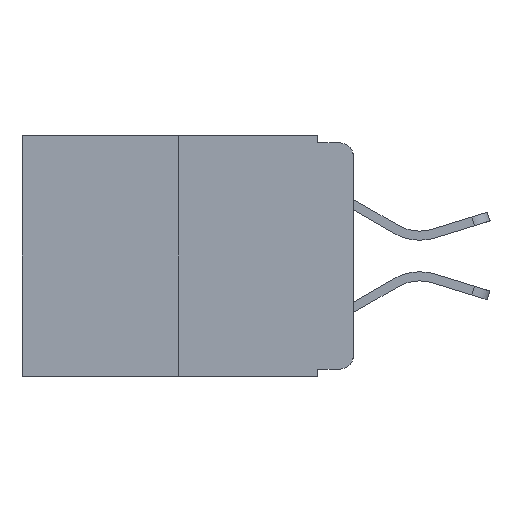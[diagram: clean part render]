
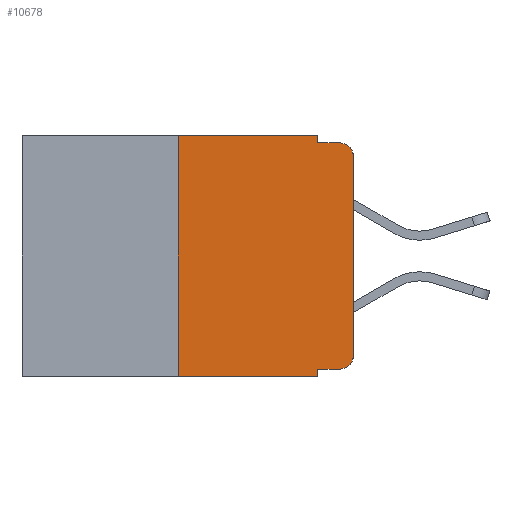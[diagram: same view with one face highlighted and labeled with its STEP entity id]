
A CAD part, left-side view. The second image highlights one B-rep face of the part: STEP entity #10678.
In plain terms, the highlighted planar face has unit normal (-1, 0, 0).
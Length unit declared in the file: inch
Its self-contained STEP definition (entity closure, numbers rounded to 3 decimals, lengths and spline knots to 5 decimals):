
#51 = ORIENTED_EDGE ( 'NONE', *, *, #3855, .T. ) ;
#233 = CARTESIAN_POINT ( 'NONE',  ( 0., 0.25, 0. ) ) ;
#453 = DIRECTION ( 'NONE',  ( -1., 0., 0. ) ) ;
#461 = VECTOR ( 'NONE', #6910, 39.37008 ) ;
#1703 = VECTOR ( 'NONE', #13378, 39.37008 ) ;
#1910 = CARTESIAN_POINT ( 'NONE',  ( 0., 0.051, 0. ) ) ;
#2035 = CARTESIAN_POINT ( 'NONE',  ( 0., 0.051, -0.333 ) ) ;
#2310 = VERTEX_POINT ( 'NONE', #12257 ) ;
#2331 = ORIENTED_EDGE ( 'NONE', *, *, #18353, .F. ) ;
#2452 = VERTEX_POINT ( 'NONE', #16747 ) ;
#2544 = ORIENTED_EDGE ( 'NONE', *, *, #15218, .F. ) ;
#2685 = EDGE_CURVE ( 'NONE', #2310, #16039, #17620, .T. ) ;
#2820 = CARTESIAN_POINT ( 'NONE',  ( 0., 0.25, -0.343 ) ) ;
#2927 = CARTESIAN_POINT ( 'NONE',  ( 0., 0.051, 0. ) ) ;
#3038 = DIRECTION ( 'NONE',  ( 0., 0., -1. ) ) ;
#3256 = ORIENTED_EDGE ( 'NONE', *, *, #7961, .T. ) ;
#3326 = AXIS2_PLACEMENT_3D ( 'NONE', #13756, #5247, #15170 ) ;
#3532 = LINE ( 'NONE', #233, #14521 ) ;
#3755 = ORIENTED_EDGE ( 'NONE', *, *, #10167, .T. ) ;
#3855 = EDGE_CURVE ( 'NONE', #5037, #9958, #14087, .T. ) ;
#3957 = ORIENTED_EDGE ( 'NONE', *, *, #10446, .F. ) ;
#4077 = EDGE_CURVE ( 'NONE', #9958, #2452, #10511, .T. ) ;
#4297 = FACE_OUTER_BOUND ( 'NONE', #16642, .T. ) ;
#4367 = CARTESIAN_POINT ( 'NONE',  ( 0., 0., -0.313 ) ) ;
#4392 = CARTESIAN_POINT ( 'NONE',  ( 0., 0.051, -0.333 ) ) ;
#4405 = ORIENTED_EDGE ( 'NONE', *, *, #6664, .F. ) ;
#4444 = DIRECTION ( 'NONE',  ( 0., 0., -1. ) ) ;
#4838 = CARTESIAN_POINT ( 'NONE',  ( 0., 0.473, -0.343 ) ) ;
#5037 = VERTEX_POINT ( 'NONE', #15895 ) ;
#5043 = LINE ( 'NONE', #18194, #461 ) ;
#5051 = LINE ( 'NONE', #14589, #12199 ) ;
#5247 = DIRECTION ( 'NONE',  ( -1., 0., 0. ) ) ;
#5394 = VERTEX_POINT ( 'NONE', #8325 ) ;
#5466 = CARTESIAN_POINT ( 'NONE',  ( 0., 0., 0. ) ) ;
#6664 = EDGE_CURVE ( 'NONE', #16112, #14730, #3532, .T. ) ;
#6910 = DIRECTION ( 'NONE',  ( 0., -1., 0. ) ) ;
#7139 = VERTEX_POINT ( 'NONE', #4392 ) ;
#7174 = AXIS2_PLACEMENT_3D ( 'NONE', #18675, #11700, #3038 ) ;
#7441 = AXIS2_PLACEMENT_3D ( 'NONE', #9296, #453, #10756 ) ;
#7761 = DIRECTION ( 'NONE',  ( 0., 0., 1. ) ) ;
#7961 = EDGE_CURVE ( 'NONE', #2452, #5394, #12495, .T. ) ;
#8060 = VERTEX_POINT ( 'NONE', #16728 ) ;
#8305 = DIRECTION ( 'NONE',  ( 0., 0., 1. ) ) ;
#8325 = CARTESIAN_POINT ( 'NONE',  ( 0., 0.02, -0.01 ) ) ;
#9296 = CARTESIAN_POINT ( 'NONE',  ( 0., 0.02, -0.313 ) ) ;
#9376 = ORIENTED_EDGE ( 'NONE', *, *, #2685, .F. ) ;
#9576 = VECTOR ( 'NONE', #12102, 39.37008 ) ;
#9850 = ORIENTED_EDGE ( 'NONE', *, *, #4077, .T. ) ;
#9958 = VERTEX_POINT ( 'NONE', #4367 ) ;
#10167 = EDGE_CURVE ( 'NONE', #16112, #8060, #13284, .T. ) ;
#10241 = PLANE ( 'NONE',  #7174 ) ;
#10446 = EDGE_CURVE ( 'NONE', #14730, #2310, #5043, .T. ) ;
#10511 = LINE ( 'NONE', #5466, #17567 ) ;
#10568 = VECTOR ( 'NONE', #4444, 39.37008 ) ;
#10678 = ADVANCED_FACE ( 'NONE', ( #4297 ), #10241, .F. ) ;
#10756 = DIRECTION ( 'NONE',  ( 0., 0., -1. ) ) ;
#11700 = DIRECTION ( 'NONE',  ( 1., 0., 0. ) ) ;
#11753 = DIRECTION ( 'NONE',  ( 0., -1., 0. ) ) ;
#12102 = DIRECTION ( 'NONE',  ( 0., 0., -1. ) ) ;
#12199 = VECTOR ( 'NONE', #11753, 39.37008 ) ;
#12223 = DIRECTION ( 'NONE',  ( 0., -1., 0. ) ) ;
#12257 = CARTESIAN_POINT ( 'NONE',  ( 0., 0.051, 0. ) ) ;
#12495 = CIRCLE ( 'NONE', #3326, 0.02 ) ;
#12933 = LINE ( 'NONE', #1910, #9576 ) ;
#13077 = VECTOR ( 'NONE', #12223, 39.37008 ) ;
#13284 = LINE ( 'NONE', #4838, #1703 ) ;
#13378 = DIRECTION ( 'NONE',  ( 0., -1., 0. ) ) ;
#13756 = CARTESIAN_POINT ( 'NONE',  ( 0., 0.02, -0.03 ) ) ;
#13778 = CARTESIAN_POINT ( 'NONE',  ( 0., 0.25, 0. ) ) ;
#13858 = ORIENTED_EDGE ( 'NONE', *, *, #17907, .T. ) ;
#14087 = CIRCLE ( 'NONE', #7441, 0.02 ) ;
#14159 = CARTESIAN_POINT ( 'NONE',  ( 0., 0.051, -0.01 ) ) ;
#14521 = VECTOR ( 'NONE', #7761, 39.37008 ) ;
#14589 = CARTESIAN_POINT ( 'NONE',  ( 0., 0.051, -0.01 ) ) ;
#14730 = VERTEX_POINT ( 'NONE', #13778 ) ;
#15170 = DIRECTION ( 'NONE',  ( 0., 0., -1. ) ) ;
#15218 = EDGE_CURVE ( 'NONE', #7139, #8060, #12933, .T. ) ;
#15895 = CARTESIAN_POINT ( 'NONE',  ( 0., 0.02, -0.333 ) ) ;
#15921 = LINE ( 'NONE', #2035, #13077 ) ;
#16039 = VERTEX_POINT ( 'NONE', #14159 ) ;
#16112 = VERTEX_POINT ( 'NONE', #2820 ) ;
#16642 = EDGE_LOOP ( 'NONE', ( #9850, #3256, #2331, #9376, #3957, #4405, #3755, #2544, #13858, #51 ) ) ;
#16728 = CARTESIAN_POINT ( 'NONE',  ( 0., 0.051, -0.343 ) ) ;
#16747 = CARTESIAN_POINT ( 'NONE',  ( 0., 0., -0.03 ) ) ;
#17567 = VECTOR ( 'NONE', #8305, 39.37008 ) ;
#17620 = LINE ( 'NONE', #2927, #10568 ) ;
#17907 = EDGE_CURVE ( 'NONE', #7139, #5037, #15921, .T. ) ;
#18194 = CARTESIAN_POINT ( 'NONE',  ( 0., 0.473, 0. ) ) ;
#18353 = EDGE_CURVE ( 'NONE', #16039, #5394, #5051, .T. ) ;
#18675 = CARTESIAN_POINT ( 'NONE',  ( 0., 0.473, 0. ) ) ;
